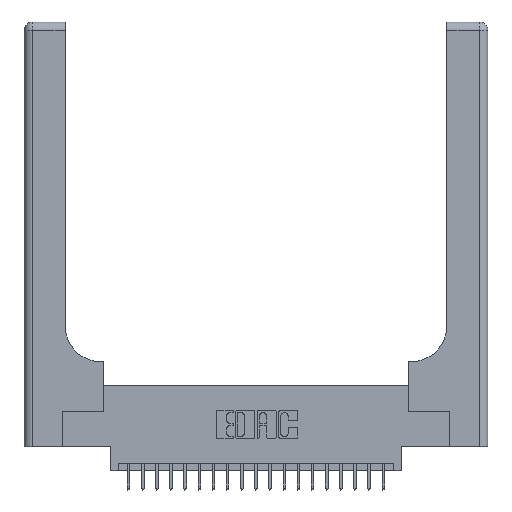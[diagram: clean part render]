
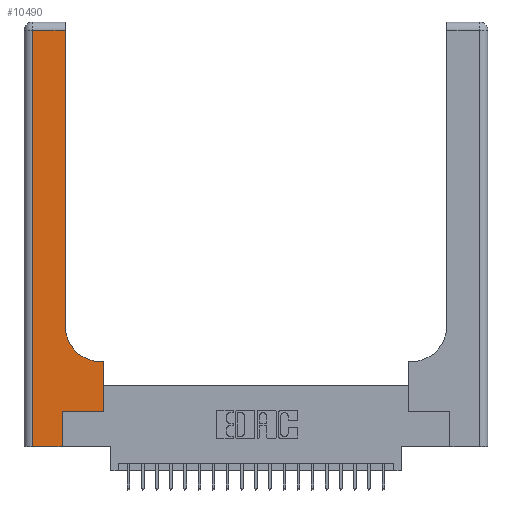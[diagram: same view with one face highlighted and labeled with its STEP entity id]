
A CAD part, top view. The second image highlights one B-rep face of the part: STEP entity #10490.
In plain terms, the highlighted planar face has unit normal (0, 0, 1).
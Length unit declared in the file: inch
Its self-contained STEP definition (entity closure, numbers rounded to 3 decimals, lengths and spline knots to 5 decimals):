
#164 = DIRECTION ( 'NONE',  ( 0., 1., 0. ) ) ;
#222 = EDGE_CURVE ( 'NONE', #11436, #5628, #18624, .T. ) ;
#353 = VECTOR ( 'NONE', #14974, 39.37008 ) ;
#727 = CARTESIAN_POINT ( 'NONE',  ( 0.5415, 0.6, 0.37 ) ) ;
#884 = EDGE_CURVE ( 'NONE', #5628, #4119, #22749, .T. ) ;
#1329 = VECTOR ( 'NONE', #2937, 39.37008 ) ;
#1427 = DIRECTION ( 'NONE',  ( 1., 0., 0. ) ) ;
#1458 = CARTESIAN_POINT ( 'NONE',  ( 0., 2.94, 0.37 ) ) ;
#1612 = CARTESIAN_POINT ( 'NONE',  ( 0.5585, 0.25, 0.37 ) ) ;
#1869 = ORIENTED_EDGE ( 'NONE', *, *, #12298, .T. ) ;
#2937 = DIRECTION ( 'NONE',  ( 0., 1., 0. ) ) ;
#2956 = VERTEX_POINT ( 'NONE', #15293 ) ;
#3159 = VECTOR ( 'NONE', #8470, 39.37008 ) ;
#3584 = ORIENTED_EDGE ( 'NONE', *, *, #20000, .T. ) ;
#4094 = EDGE_LOOP ( 'NONE', ( #8830, #11906, #21223, #20459, #3584, #17681, #11122, #9621, #1869 ) ) ;
#4119 = VERTEX_POINT ( 'NONE', #727 ) ;
#4511 = DIRECTION ( 'NONE',  ( 0., -1., 0. ) ) ;
#4564 = CARTESIAN_POINT ( 'NONE',  ( 0.5585, 0.6, 0.37 ) ) ;
#4999 = LINE ( 'NONE', #1458, #17231 ) ;
#5439 = DIRECTION ( 'NONE',  ( 0., 0., -1. ) ) ;
#5628 = VERTEX_POINT ( 'NONE', #4564 ) ;
#6184 = LINE ( 'NONE', #6298, #13422 ) ;
#6298 = CARTESIAN_POINT ( 'NONE',  ( 0.06, 3., 0.37 ) ) ;
#6479 = LINE ( 'NONE', #18825, #1329 ) ;
#7980 = VERTEX_POINT ( 'NONE', #15352 ) ;
#8026 = EDGE_CURVE ( 'NONE', #8965, #22667, #4999, .T. ) ;
#8245 = CARTESIAN_POINT ( 'NONE',  ( 0., 0., 0.37 ) ) ;
#8470 = DIRECTION ( 'NONE',  ( 1., 0., 0. ) ) ;
#8722 = VERTEX_POINT ( 'NONE', #15173 ) ;
#8830 = ORIENTED_EDGE ( 'NONE', *, *, #17792, .T. ) ;
#8965 = VERTEX_POINT ( 'NONE', #9451 ) ;
#9451 = CARTESIAN_POINT ( 'NONE',  ( 0.2915, 2.94, 0.37 ) ) ;
#9621 = ORIENTED_EDGE ( 'NONE', *, *, #884, .T. ) ;
#9859 = AXIS2_PLACEMENT_3D ( 'NONE', #16010, #5439, #1427 ) ;
#10226 = VECTOR ( 'NONE', #164, 39.37008 ) ;
#10237 = VECTOR ( 'NONE', #12093, 39.37008 ) ;
#10490 = ADVANCED_FACE ( 'NONE', ( #14652 ), #21379, .F. ) ;
#10710 = EDGE_CURVE ( 'NONE', #22667, #2956, #6184, .T. ) ;
#11122 = ORIENTED_EDGE ( 'NONE', *, *, #222, .T. ) ;
#11436 = VERTEX_POINT ( 'NONE', #1612 ) ;
#11906 = ORIENTED_EDGE ( 'NONE', *, *, #8026, .T. ) ;
#12074 = LINE ( 'NONE', #12312, #19794 ) ;
#12093 = DIRECTION ( 'NONE',  ( -1., 0., 0. ) ) ;
#12298 = EDGE_CURVE ( 'NONE', #4119, #8722, #20062, .T. ) ;
#12312 = CARTESIAN_POINT ( 'NONE',  ( 0.2915, 3., 0.37 ) ) ;
#13422 = VECTOR ( 'NONE', #4511, 39.37008 ) ;
#13804 = DIRECTION ( 'NONE',  ( -1., 0., 0. ) ) ;
#14111 = CARTESIAN_POINT ( 'NONE',  ( 0.2915, 0.6, 0.37 ) ) ;
#14171 = DIRECTION ( 'NONE',  ( 0., 0., -1. ) ) ;
#14524 = CARTESIAN_POINT ( 'NONE',  ( 0.5585, 0.25, 0.37 ) ) ;
#14652 = FACE_OUTER_BOUND ( 'NONE', #4094, .T. ) ;
#14974 = DIRECTION ( 'NONE',  ( 1., 0., 0. ) ) ;
#15173 = CARTESIAN_POINT ( 'NONE',  ( 0.2915, 0.85, 0.37 ) ) ;
#15293 = CARTESIAN_POINT ( 'NONE',  ( 0.06, 0., 0.37 ) ) ;
#15352 = CARTESIAN_POINT ( 'NONE',  ( 0.269, 0., 0.37 ) ) ;
#15923 = CARTESIAN_POINT ( 'NONE',  ( 0., 3., 0.37 ) ) ;
#16010 = CARTESIAN_POINT ( 'NONE',  ( 0.5415, 0.85, 0.37 ) ) ;
#17231 = VECTOR ( 'NONE', #13804, 39.37008 ) ;
#17459 = LINE ( 'NONE', #8245, #3159 ) ;
#17681 = ORIENTED_EDGE ( 'NONE', *, *, #22780, .T. ) ;
#17792 = EDGE_CURVE ( 'NONE', #8722, #8965, #12074, .T. ) ;
#17805 = VERTEX_POINT ( 'NONE', #21064 ) ;
#18039 = CARTESIAN_POINT ( 'NONE',  ( 0.06, 2.94, 0.37 ) ) ;
#18188 = EDGE_CURVE ( 'NONE', #2956, #7980, #17459, .T. ) ;
#18624 = LINE ( 'NONE', #14524, #10226 ) ;
#18825 = CARTESIAN_POINT ( 'NONE',  ( 0.269, 0., 0.37 ) ) ;
#19794 = VECTOR ( 'NONE', #22725, 39.37008 ) ;
#20000 = EDGE_CURVE ( 'NONE', #7980, #17805, #6479, .T. ) ;
#20062 = CIRCLE ( 'NONE', #9859, 0.25 ) ;
#20459 = ORIENTED_EDGE ( 'NONE', *, *, #18188, .T. ) ;
#20529 = CARTESIAN_POINT ( 'NONE',  ( 0.269, 0.25, 0.37 ) ) ;
#21064 = CARTESIAN_POINT ( 'NONE',  ( 0.269, 0.25, 0.37 ) ) ;
#21223 = ORIENTED_EDGE ( 'NONE', *, *, #10710, .T. ) ;
#21379 = PLANE ( 'NONE',  #21421 ) ;
#21421 = AXIS2_PLACEMENT_3D ( 'NONE', #15923, #14171, #21854 ) ;
#21854 = DIRECTION ( 'NONE',  ( -1., 0., 0. ) ) ;
#22064 = LINE ( 'NONE', #20529, #353 ) ;
#22667 = VERTEX_POINT ( 'NONE', #18039 ) ;
#22725 = DIRECTION ( 'NONE',  ( 0., 1., 0. ) ) ;
#22749 = LINE ( 'NONE', #14111, #10237 ) ;
#22780 = EDGE_CURVE ( 'NONE', #17805, #11436, #22064, .T. ) ;
